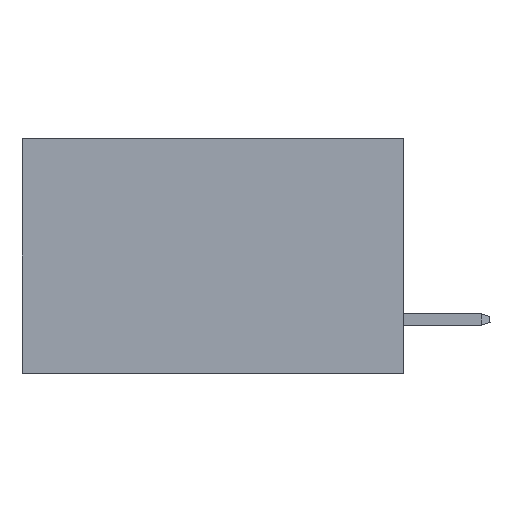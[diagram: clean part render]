
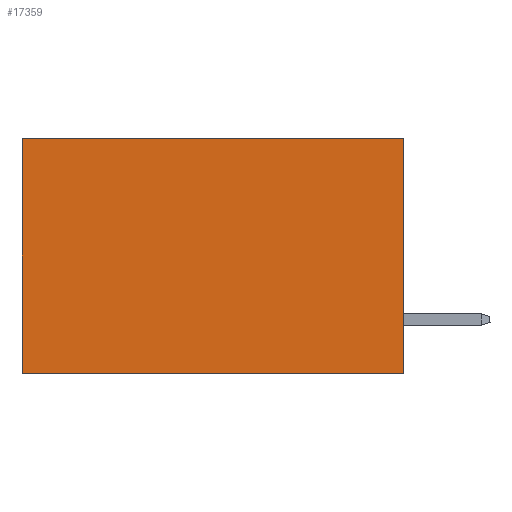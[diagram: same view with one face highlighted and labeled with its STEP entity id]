
A CAD part, left-side view. The second image highlights one B-rep face of the part: STEP entity #17359.
In plain terms, the highlighted planar face has unit normal (-1, 0, 0).
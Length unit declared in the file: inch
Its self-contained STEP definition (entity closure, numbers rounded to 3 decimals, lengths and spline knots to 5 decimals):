
#935 = EDGE_CURVE ( 'NONE', #8033, #6128, #12424, .T. ) ;
#2120 = AXIS2_PLACEMENT_3D ( 'NONE', #2852, #17805, #5481 ) ;
#2376 = CARTESIAN_POINT ( 'NONE',  ( 0.2875, 0.6, 0. ) ) ;
#2517 = EDGE_LOOP ( 'NONE', ( #13441, #15039, #3310, #12198 ) ) ;
#2638 = DIRECTION ( 'NONE',  ( 0., 0., -1. ) ) ;
#2852 = CARTESIAN_POINT ( 'NONE',  ( 0.2875, 0., 0. ) ) ;
#2977 = VECTOR ( 'NONE', #7920, 39.37008 ) ;
#3310 = ORIENTED_EDGE ( 'NONE', *, *, #12725, .F. ) ;
#3686 = CARTESIAN_POINT ( 'NONE',  ( 0.2875, 0., 0. ) ) ;
#3834 = CARTESIAN_POINT ( 'NONE',  ( 0.2875, 0., 0. ) ) ;
#4781 = VECTOR ( 'NONE', #10723, 39.37008 ) ;
#4840 = EDGE_CURVE ( 'NONE', #5498, #6128, #9514, .T. ) ;
#5481 = DIRECTION ( 'NONE',  ( 0., 0., -1. ) ) ;
#5498 = VERTEX_POINT ( 'NONE', #11272 ) ;
#6128 = VERTEX_POINT ( 'NONE', #8825 ) ;
#6145 = VERTEX_POINT ( 'NONE', #9004 ) ;
#7920 = DIRECTION ( 'NONE',  ( 0., 1., 0. ) ) ;
#8033 = VERTEX_POINT ( 'NONE', #11946 ) ;
#8334 = DIRECTION ( 'NONE',  ( 0., 0., -1. ) ) ;
#8352 = FACE_OUTER_BOUND ( 'NONE', #2517, .T. ) ;
#8825 = CARTESIAN_POINT ( 'NONE',  ( 0.2875, 0.6, -0.37 ) ) ;
#9004 = CARTESIAN_POINT ( 'NONE',  ( 0.2875, 0., 0. ) ) ;
#9514 = LINE ( 'NONE', #2376, #16891 ) ;
#10723 = DIRECTION ( 'NONE',  ( 0., 1., 0. ) ) ;
#11272 = CARTESIAN_POINT ( 'NONE',  ( 0.2875, 0.6, 0. ) ) ;
#11946 = CARTESIAN_POINT ( 'NONE',  ( 0.2875, 0., -0.37 ) ) ;
#12198 = ORIENTED_EDGE ( 'NONE', *, *, #15762, .T. ) ;
#12424 = LINE ( 'NONE', #13754, #2977 ) ;
#12725 = EDGE_CURVE ( 'NONE', #6145, #8033, #13636, .T. ) ;
#13441 = ORIENTED_EDGE ( 'NONE', *, *, #4840, .T. ) ;
#13636 = LINE ( 'NONE', #3834, #17060 ) ;
#13754 = CARTESIAN_POINT ( 'NONE',  ( 0.2875, 0., -0.37 ) ) ;
#13836 = PLANE ( 'NONE',  #2120 ) ;
#15039 = ORIENTED_EDGE ( 'NONE', *, *, #935, .F. ) ;
#15762 = EDGE_CURVE ( 'NONE', #6145, #5498, #17541, .T. ) ;
#16891 = VECTOR ( 'NONE', #2638, 39.37008 ) ;
#17060 = VECTOR ( 'NONE', #8334, 39.37008 ) ;
#17359 = ADVANCED_FACE ( 'NONE', ( #8352 ), #13836, .F. ) ;
#17541 = LINE ( 'NONE', #3686, #4781 ) ;
#17805 = DIRECTION ( 'NONE',  ( 1., 0., 0. ) ) ;
